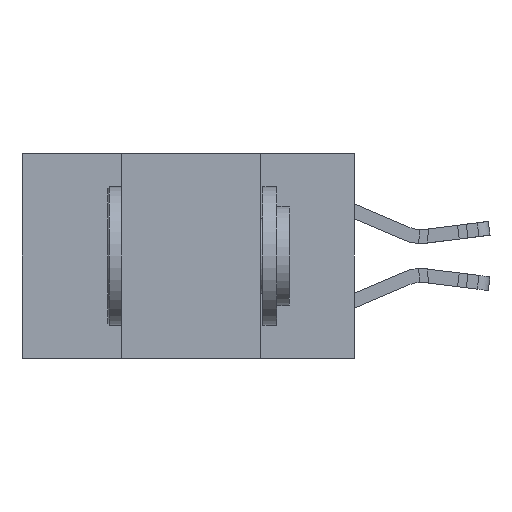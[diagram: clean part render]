
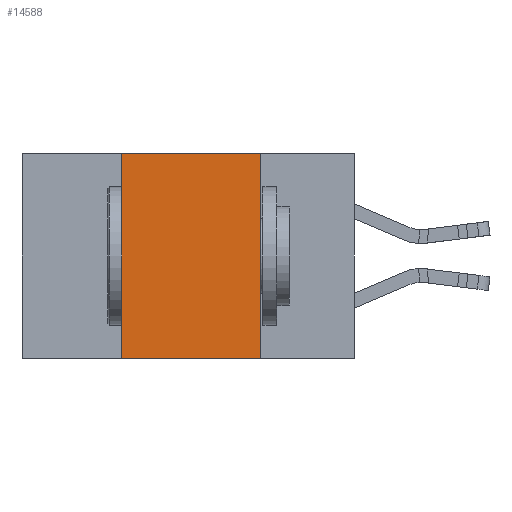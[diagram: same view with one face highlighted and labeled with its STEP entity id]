
A CAD part, left-side view. The second image highlights one B-rep face of the part: STEP entity #14588.
In plain terms, the highlighted planar face has unit normal (-1, 0, 0).
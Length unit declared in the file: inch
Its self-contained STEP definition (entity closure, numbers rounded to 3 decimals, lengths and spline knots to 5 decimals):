
#288 = ORIENTED_EDGE ( 'NONE', *, *, #16619, .F. ) ;
#558 = CARTESIAN_POINT ( 'NONE',  ( 0., 0.6, -0.37 ) ) ;
#810 = LINE ( 'NONE', #558, #20637 ) ;
#1183 = VERTEX_POINT ( 'NONE', #17974 ) ;
#1468 = CARTESIAN_POINT ( 'NONE',  ( 0., 0.42, 0. ) ) ;
#1671 = ORIENTED_EDGE ( 'NONE', *, *, #25618, .F. ) ;
#2548 = CARTESIAN_POINT ( 'NONE',  ( 0., 0.17, -0.37 ) ) ;
#4809 = ORIENTED_EDGE ( 'NONE', *, *, #19071, .F. ) ;
#5070 = AXIS2_PLACEMENT_3D ( 'NONE', #7328, #17366, #19751 ) ;
#5113 = DIRECTION ( 'NONE',  ( 0., 0., -1. ) ) ;
#5386 = CARTESIAN_POINT ( 'NONE',  ( 0., 0.17, -0.37 ) ) ;
#6977 = ORIENTED_EDGE ( 'NONE', *, *, #11518, .T. ) ;
#7328 = CARTESIAN_POINT ( 'NONE',  ( 0., 0.6, 0. ) ) ;
#8957 = VERTEX_POINT ( 'NONE', #1468 ) ;
#9182 = VECTOR ( 'NONE', #9305, 39.37008 ) ;
#9305 = DIRECTION ( 'NONE',  ( 0., -1., 0. ) ) ;
#9312 = FACE_OUTER_BOUND ( 'NONE', #9494, .T. ) ;
#9494 = EDGE_LOOP ( 'NONE', ( #1671, #4809, #288, #6977 ) ) ;
#11518 = EDGE_CURVE ( 'NONE', #1183, #23275, #810, .T. ) ;
#12333 = VECTOR ( 'NONE', #5113, 39.37008 ) ;
#13999 = CARTESIAN_POINT ( 'NONE',  ( 0., 0.42, -0.37 ) ) ;
#14173 = CARTESIAN_POINT ( 'NONE',  ( 0., 0.17, 0. ) ) ;
#14588 = ADVANCED_FACE ( 'NONE', ( #9312 ), #21593, .F. ) ;
#15520 = LINE ( 'NONE', #19209, #9182 ) ;
#15713 = LINE ( 'NONE', #5386, #12333 ) ;
#16232 = LINE ( 'NONE', #13999, #22474 ) ;
#16619 = EDGE_CURVE ( 'NONE', #1183, #8957, #16232, .T. ) ;
#17366 = DIRECTION ( 'NONE',  ( 1., 0., 0. ) ) ;
#17974 = CARTESIAN_POINT ( 'NONE',  ( 0., 0.42, -0.37 ) ) ;
#19071 = EDGE_CURVE ( 'NONE', #8957, #22425, #15520, .T. ) ;
#19209 = CARTESIAN_POINT ( 'NONE',  ( 0., 0.6, 0. ) ) ;
#19751 = DIRECTION ( 'NONE',  ( 0., 0., -1. ) ) ;
#20637 = VECTOR ( 'NONE', #23036, 39.37008 ) ;
#21593 = PLANE ( 'NONE',  #5070 ) ;
#22425 = VERTEX_POINT ( 'NONE', #14173 ) ;
#22474 = VECTOR ( 'NONE', #24031, 39.37008 ) ;
#23036 = DIRECTION ( 'NONE',  ( 0., -1., 0. ) ) ;
#23275 = VERTEX_POINT ( 'NONE', #2548 ) ;
#24031 = DIRECTION ( 'NONE',  ( 0., 0., 1. ) ) ;
#25618 = EDGE_CURVE ( 'NONE', #22425, #23275, #15713, .T. ) ;
